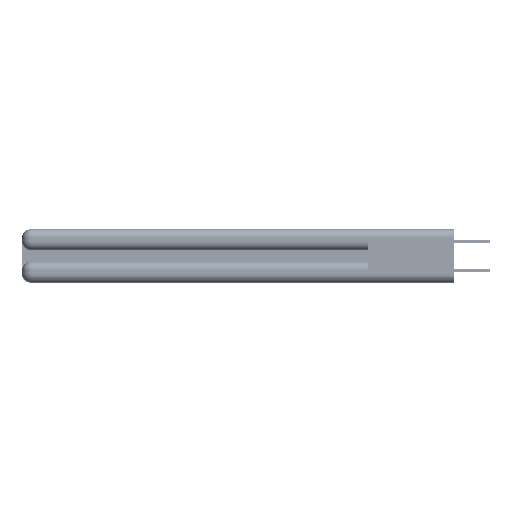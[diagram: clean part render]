
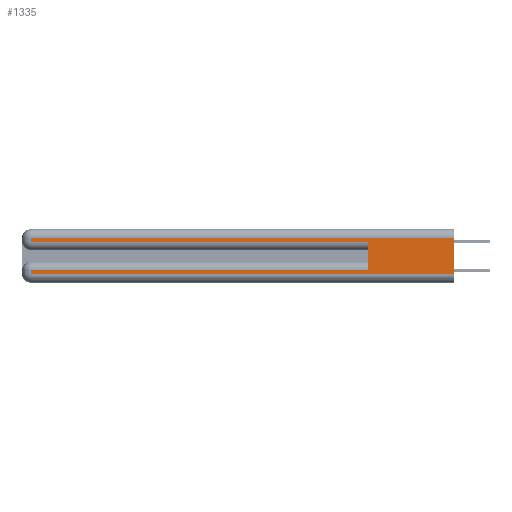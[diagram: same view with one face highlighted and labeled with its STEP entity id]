
A CAD part, left-side view. The second image highlights one B-rep face of the part: STEP entity #1335.
In plain terms, the highlighted planar face has unit normal (-1, 0, 0).
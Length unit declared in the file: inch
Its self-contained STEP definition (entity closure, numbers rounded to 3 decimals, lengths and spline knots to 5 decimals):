
#265 = LINE ( 'NONE', #3306, #47119 ) ;
#909 = VECTOR ( 'NONE', #4341, 39.37008 ) ;
#1335 = ADVANCED_FACE ( 'NONE', ( #40889 ), #15228, .F. ) ;
#1497 = CARTESIAN_POINT ( 'NONE',  ( 0., 2.94, 0.06 ) ) ;
#1895 = CARTESIAN_POINT ( 'NONE',  ( 0., 0., 0.285 ) ) ;
#2144 = LINE ( 'NONE', #37650, #909 ) ;
#3298 = VECTOR ( 'NONE', #38764, 39.37008 ) ;
#3306 = CARTESIAN_POINT ( 'NONE',  ( 0., 0., 0.31 ) ) ;
#3938 = VERTEX_POINT ( 'NONE', #44412 ) ;
#4341 = DIRECTION ( 'NONE',  ( 0., 1., 0. ) ) ;
#5158 = DIRECTION ( 'NONE',  ( 0., -1., 0. ) ) ;
#5178 = LINE ( 'NONE', #5435, #40419 ) ;
#5435 = CARTESIAN_POINT ( 'NONE',  ( 0., 2.94, 0.37 ) ) ;
#5920 = VECTOR ( 'NONE', #5158, 39.37008 ) ;
#7687 = ORIENTED_EDGE ( 'NONE', *, *, #27341, .F. ) ;
#9685 = DIRECTION ( 'NONE',  ( 0., 0., -1. ) ) ;
#10165 = EDGE_CURVE ( 'NONE', #19940, #10693, #265, .T. ) ;
#10532 = CARTESIAN_POINT ( 'NONE',  ( 0., 0., 0.06 ) ) ;
#10693 = VERTEX_POINT ( 'NONE', #43821 ) ;
#11233 = DIRECTION ( 'NONE',  ( 0., 1., 0. ) ) ;
#11236 = DIRECTION ( 'NONE',  ( 0., 0., -1. ) ) ;
#11894 = DIRECTION ( 'NONE',  ( 0., 0., 1. ) ) ;
#12770 = ORIENTED_EDGE ( 'NONE', *, *, #10165, .T. ) ;
#13115 = LINE ( 'NONE', #1895, #3298 ) ;
#13927 = CARTESIAN_POINT ( 'NONE',  ( 0., 0.6, 0.285 ) ) ;
#15039 = CARTESIAN_POINT ( 'NONE',  ( 0., 0., 0.31 ) ) ;
#15108 = VERTEX_POINT ( 'NONE', #1497 ) ;
#15228 = PLANE ( 'NONE',  #38508 ) ;
#17840 = EDGE_CURVE ( 'NONE', #10693, #43741, #22441, .T. ) ;
#18494 = CARTESIAN_POINT ( 'NONE',  ( 0., 0., 0.37 ) ) ;
#18598 = LINE ( 'NONE', #38267, #5920 ) ;
#19940 = VERTEX_POINT ( 'NONE', #15039 ) ;
#20066 = ORIENTED_EDGE ( 'NONE', *, *, #40986, .F. ) ;
#21104 = CARTESIAN_POINT ( 'NONE',  ( 0., 0.6, 0.085 ) ) ;
#21989 = EDGE_LOOP ( 'NONE', ( #20066, #12770, #23754, #27874, #7687, #38526, #33496, #44484 ) ) ;
#22441 = LINE ( 'NONE', #41549, #37441 ) ;
#22728 = EDGE_CURVE ( 'NONE', #15108, #43895, #18598, .T. ) ;
#23674 = CARTESIAN_POINT ( 'NONE',  ( 0., 0., 0.37 ) ) ;
#23754 = ORIENTED_EDGE ( 'NONE', *, *, #17840, .T. ) ;
#27341 = EDGE_CURVE ( 'NONE', #39171, #35195, #35874, .T. ) ;
#27874 = ORIENTED_EDGE ( 'NONE', *, *, #29583, .T. ) ;
#27986 = EDGE_CURVE ( 'NONE', #3938, #15108, #5178, .T. ) ;
#28467 = LINE ( 'NONE', #23674, #30736 ) ;
#29583 = EDGE_CURVE ( 'NONE', #43741, #35195, #13115, .T. ) ;
#30736 = VECTOR ( 'NONE', #45536, 39.37008 ) ;
#32403 = VECTOR ( 'NONE', #11894, 39.37008 ) ;
#33496 = ORIENTED_EDGE ( 'NONE', *, *, #27986, .T. ) ;
#35195 = VERTEX_POINT ( 'NONE', #13927 ) ;
#35874 = LINE ( 'NONE', #44783, #32403 ) ;
#37214 = DIRECTION ( 'NONE',  ( 1., 0., 0. ) ) ;
#37441 = VECTOR ( 'NONE', #42180, 39.37008 ) ;
#37650 = CARTESIAN_POINT ( 'NONE',  ( 0., 0., 0.085 ) ) ;
#38267 = CARTESIAN_POINT ( 'NONE',  ( 0., 0., 0.06 ) ) ;
#38508 = AXIS2_PLACEMENT_3D ( 'NONE', #18494, #37214, #11236 ) ;
#38526 = ORIENTED_EDGE ( 'NONE', *, *, #46390, .T. ) ;
#38764 = DIRECTION ( 'NONE',  ( 0., -1., 0. ) ) ;
#39171 = VERTEX_POINT ( 'NONE', #21104 ) ;
#40419 = VECTOR ( 'NONE', #9685, 39.37008 ) ;
#40889 = FACE_OUTER_BOUND ( 'NONE', #21989, .T. ) ;
#40986 = EDGE_CURVE ( 'NONE', #19940, #43895, #28467, .T. ) ;
#41549 = CARTESIAN_POINT ( 'NONE',  ( 0., 2.94, 0.37 ) ) ;
#42180 = DIRECTION ( 'NONE',  ( 0., 0., -1. ) ) ;
#43741 = VERTEX_POINT ( 'NONE', #47106 ) ;
#43821 = CARTESIAN_POINT ( 'NONE',  ( 0., 2.94, 0.31 ) ) ;
#43895 = VERTEX_POINT ( 'NONE', #10532 ) ;
#44412 = CARTESIAN_POINT ( 'NONE',  ( 0., 2.94, 0.085 ) ) ;
#44484 = ORIENTED_EDGE ( 'NONE', *, *, #22728, .T. ) ;
#44783 = CARTESIAN_POINT ( 'NONE',  ( 0., 0.6, 0.145 ) ) ;
#45536 = DIRECTION ( 'NONE',  ( 0., 0., -1. ) ) ;
#46390 = EDGE_CURVE ( 'NONE', #39171, #3938, #2144, .T. ) ;
#47106 = CARTESIAN_POINT ( 'NONE',  ( 0., 2.94, 0.285 ) ) ;
#47119 = VECTOR ( 'NONE', #11233, 39.37008 ) ;
